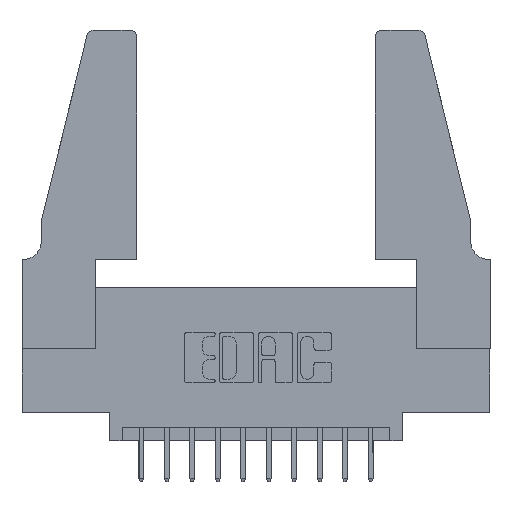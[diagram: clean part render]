
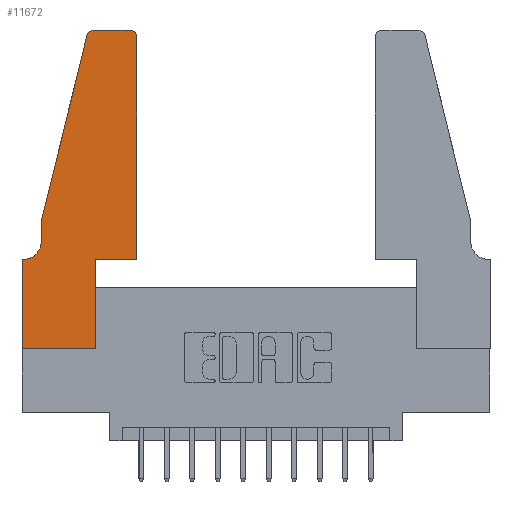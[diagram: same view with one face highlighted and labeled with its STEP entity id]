
A CAD part, top view. The second image highlights one B-rep face of the part: STEP entity #11672.
In plain terms, the highlighted planar face has unit normal (0, 0, 1).
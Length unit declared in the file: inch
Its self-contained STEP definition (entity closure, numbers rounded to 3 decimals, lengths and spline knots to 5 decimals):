
#74 = CARTESIAN_POINT ( 'NONE',  ( 0., 0.35, 0.37 ) ) ;
#437 = LINE ( 'NONE', #6807, #9568 ) ;
#640 = ORIENTED_EDGE ( 'NONE', *, *, #10970, .T. ) ;
#1063 = DIRECTION ( 'NONE',  ( -1., 0., 0. ) ) ;
#1066 = DIRECTION ( 'NONE',  ( 0., 1., 0. ) ) ;
#1078 = CARTESIAN_POINT ( 'NONE',  ( 0.4205, 1.25, 0.37 ) ) ;
#1537 = CARTESIAN_POINT ( 'NONE',  ( 0., 0.35, 0.37 ) ) ;
#1620 = DIRECTION ( 'NONE',  ( 1., 0., 0. ) ) ;
#1719 = CIRCLE ( 'NONE', #12026, 0.03 ) ;
#1893 = CARTESIAN_POINT ( 'NONE',  ( 0., 0., 0.37 ) ) ;
#1933 = ORIENTED_EDGE ( 'NONE', *, *, #10245, .T. ) ;
#2166 = VERTEX_POINT ( 'NONE', #1078 ) ;
#2173 = CARTESIAN_POINT ( 'NONE',  ( 0., 0., 0.37 ) ) ;
#2209 = DIRECTION ( 'NONE',  ( -0.239, -0.971, 0. ) ) ;
#2392 = CARTESIAN_POINT ( 'NONE',  ( 0.0755, 0.35, 0.37 ) ) ;
#2428 = CARTESIAN_POINT ( 'NONE',  ( 0.0055, 0.42, 0.37 ) ) ;
#2525 = CIRCLE ( 'NONE', #3151, 0.07 ) ;
#2692 = CARTESIAN_POINT ( 'NONE',  ( 0.4505, 0.35, 0.37 ) ) ;
#2796 = EDGE_CURVE ( 'NONE', #2166, #4342, #437, .T. ) ;
#2808 = VECTOR ( 'NONE', #10201, 39.37008 ) ;
#2969 = DIRECTION ( 'NONE',  ( 0., -1., 0. ) ) ;
#2997 = LINE ( 'NONE', #14315, #6367 ) ;
#3151 = AXIS2_PLACEMENT_3D ( 'NONE', #2428, #5827, #6960 ) ;
#3390 = VECTOR ( 'NONE', #4857, 39.37008 ) ;
#3683 = VERTEX_POINT ( 'NONE', #11884 ) ;
#3755 = VERTEX_POINT ( 'NONE', #11267 ) ;
#3878 = LINE ( 'NONE', #8310, #12661 ) ;
#3904 = EDGE_CURVE ( 'NONE', #7706, #8938, #2525, .T. ) ;
#3998 = DIRECTION ( 'NONE',  ( 0., 1., 0. ) ) ;
#4320 = CARTESIAN_POINT ( 'NONE',  ( 0.25487, 1.22718, 0.37 ) ) ;
#4342 = VERTEX_POINT ( 'NONE', #6469 ) ;
#4490 = CARTESIAN_POINT ( 'NONE',  ( 0.0055, 0.35, 0.37 ) ) ;
#4574 = ORIENTED_EDGE ( 'NONE', *, *, #13127, .T. ) ;
#4650 = CARTESIAN_POINT ( 'NONE',  ( 0.4205, 1.22, 0.37 ) ) ;
#4857 = DIRECTION ( 'NONE',  ( 1., 0., 0. ) ) ;
#4867 = DIRECTION ( 'NONE',  ( 1., 0., 0. ) ) ;
#5041 = DIRECTION ( 'NONE',  ( 0., 0., 1. ) ) ;
#5345 = FACE_OUTER_BOUND ( 'NONE', #13791, .T. ) ;
#5365 = ORIENTED_EDGE ( 'NONE', *, *, #12295, .T. ) ;
#5546 = VERTEX_POINT ( 'NONE', #1893 ) ;
#5720 = DIRECTION ( 'NONE',  ( 1., 0., 0. ) ) ;
#5827 = DIRECTION ( 'NONE',  ( 0., 0., -1. ) ) ;
#5864 = AXIS2_PLACEMENT_3D ( 'NONE', #4650, #8052, #5720 ) ;
#5968 = EDGE_CURVE ( 'NONE', #3683, #7706, #3878, .T. ) ;
#6176 = VERTEX_POINT ( 'NONE', #4320 ) ;
#6322 = EDGE_CURVE ( 'NONE', #5546, #3755, #8619, .T. ) ;
#6349 = CARTESIAN_POINT ( 'NONE',  ( 0.0755, 0.42, 0.37 ) ) ;
#6367 = VECTOR ( 'NONE', #2969, 39.37008 ) ;
#6454 = LINE ( 'NONE', #12897, #9235 ) ;
#6469 = CARTESIAN_POINT ( 'NONE',  ( 0.284, 1.25, 0.37 ) ) ;
#6672 = DIRECTION ( 'NONE',  ( 1., 0., 0. ) ) ;
#6807 = CARTESIAN_POINT ( 'NONE',  ( 0.2605, 1.25, 0.37 ) ) ;
#6903 = ORIENTED_EDGE ( 'NONE', *, *, #3904, .T. ) ;
#6960 = DIRECTION ( 'NONE',  ( -1., 0., 0. ) ) ;
#7084 = LINE ( 'NONE', #8262, #3390 ) ;
#7107 = EDGE_CURVE ( 'NONE', #3755, #8993, #12812, .T. ) ;
#7408 = VERTEX_POINT ( 'NONE', #9304 ) ;
#7597 = CARTESIAN_POINT ( 'NONE',  ( 0.0755, 0.5, 0.37 ) ) ;
#7607 = EDGE_CURVE ( 'NONE', #4342, #6176, #1719, .T. ) ;
#7706 = VERTEX_POINT ( 'NONE', #6349 ) ;
#8052 = DIRECTION ( 'NONE',  ( 0., 0., 1. ) ) ;
#8228 = ORIENTED_EDGE ( 'NONE', *, *, #7607, .T. ) ;
#8262 = CARTESIAN_POINT ( 'NONE',  ( 0.4505, 0.35, 0.37 ) ) ;
#8310 = CARTESIAN_POINT ( 'NONE',  ( 0.0755, 0.5, 0.37 ) ) ;
#8365 = DIRECTION ( 'NONE',  ( 0., 0., 1. ) ) ;
#8619 = LINE ( 'NONE', #2173, #12134 ) ;
#8803 = LINE ( 'NONE', #2392, #2808 ) ;
#8938 = VERTEX_POINT ( 'NONE', #4490 ) ;
#8993 = VERTEX_POINT ( 'NONE', #13371 ) ;
#9079 = CIRCLE ( 'NONE', #5864, 0.03 ) ;
#9170 = AXIS2_PLACEMENT_3D ( 'NONE', #1537, #8365, #4867 ) ;
#9235 = VECTOR ( 'NONE', #3998, 39.37008 ) ;
#9304 = CARTESIAN_POINT ( 'NONE',  ( 0.4505, 1.22, 0.37 ) ) ;
#9568 = VECTOR ( 'NONE', #1063, 39.37008 ) ;
#9971 = ORIENTED_EDGE ( 'NONE', *, *, #10480, .T. ) ;
#10201 = DIRECTION ( 'NONE',  ( -1., 0., 0. ) ) ;
#10245 = EDGE_CURVE ( 'NONE', #7408, #2166, #9079, .T. ) ;
#10386 = ORIENTED_EDGE ( 'NONE', *, *, #14062, .T. ) ;
#10480 = EDGE_CURVE ( 'NONE', #12247, #7408, #6454, .T. ) ;
#10865 = VECTOR ( 'NONE', #1066, 39.37008 ) ;
#10970 = EDGE_CURVE ( 'NONE', #6176, #3683, #13290, .T. ) ;
#11200 = ORIENTED_EDGE ( 'NONE', *, *, #2796, .T. ) ;
#11267 = CARTESIAN_POINT ( 'NONE',  ( 0.2865, 0., 0.37 ) ) ;
#11335 = ORIENTED_EDGE ( 'NONE', *, *, #6322, .T. ) ;
#11396 = VERTEX_POINT ( 'NONE', #74 ) ;
#11526 = DIRECTION ( 'NONE',  ( 0., -1., 0. ) ) ;
#11586 = PLANE ( 'NONE',  #9170 ) ;
#11672 = ADVANCED_FACE ( 'NONE', ( #5345 ), #11586, .T. ) ;
#11773 = CARTESIAN_POINT ( 'NONE',  ( 0.284, 1.22, 0.37 ) ) ;
#11884 = CARTESIAN_POINT ( 'NONE',  ( 0.0755, 0.5, 0.37 ) ) ;
#12026 = AXIS2_PLACEMENT_3D ( 'NONE', #11773, #5041, #1620 ) ;
#12134 = VECTOR ( 'NONE', #6672, 39.37008 ) ;
#12247 = VERTEX_POINT ( 'NONE', #2692 ) ;
#12295 = EDGE_CURVE ( 'NONE', #8993, #12247, #7084, .T. ) ;
#12661 = VECTOR ( 'NONE', #11526, 39.37008 ) ;
#12812 = LINE ( 'NONE', #14428, #10865 ) ;
#12897 = CARTESIAN_POINT ( 'NONE',  ( 0.4505, 0.35, 0.37 ) ) ;
#13069 = ORIENTED_EDGE ( 'NONE', *, *, #5968, .T. ) ;
#13095 = VECTOR ( 'NONE', #2209, 39.37008 ) ;
#13127 = EDGE_CURVE ( 'NONE', #11396, #5546, #2997, .T. ) ;
#13290 = LINE ( 'NONE', #7597, #13095 ) ;
#13371 = CARTESIAN_POINT ( 'NONE',  ( 0.2865, 0.35, 0.37 ) ) ;
#13791 = EDGE_LOOP ( 'NONE', ( #11200, #8228, #640, #13069, #6903, #10386, #4574, #11335, #13861, #5365, #9971, #1933 ) ) ;
#13861 = ORIENTED_EDGE ( 'NONE', *, *, #7107, .T. ) ;
#14062 = EDGE_CURVE ( 'NONE', #8938, #11396, #8803, .T. ) ;
#14315 = CARTESIAN_POINT ( 'NONE',  ( 0., 0., 0.37 ) ) ;
#14428 = CARTESIAN_POINT ( 'NONE',  ( 0.2865, 0.35, 0.37 ) ) ;
